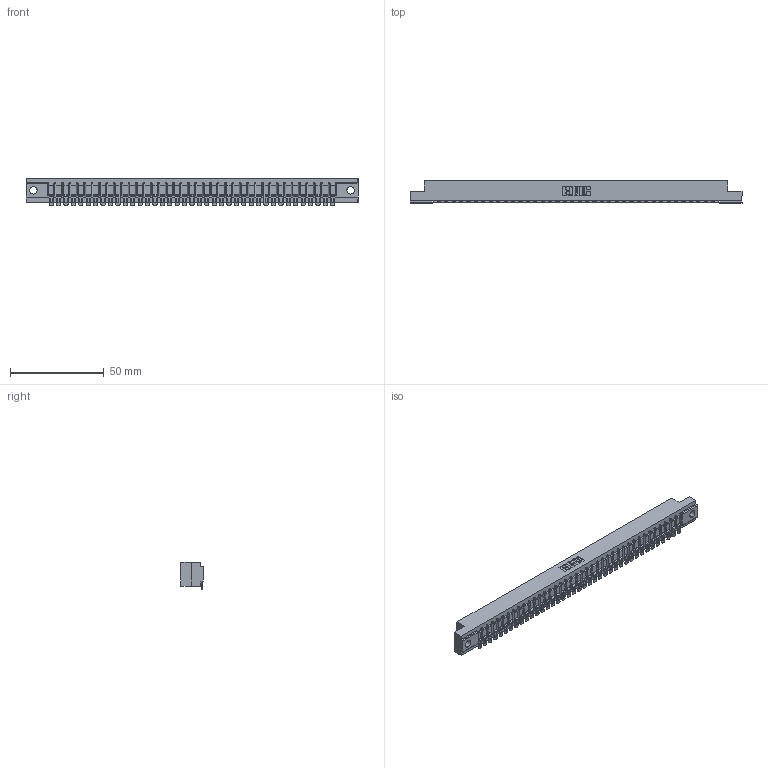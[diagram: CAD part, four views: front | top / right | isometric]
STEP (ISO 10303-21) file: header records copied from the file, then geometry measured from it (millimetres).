
FILE_DESCRIPTION (( 'STEP AP203' ), '1' );
FILE_NAME ('357-039-454-104.STEP', '2020-10-03T04:32:03', ( '' ), ( '' ), 'SwSTEP 2.0', 'SolidWorks 2020', '' );
FILE_SCHEMA (( 'CONFIG_CONTROL_DESIGN' ));
Length unit declared in the file: inch
Products named in the file (3): 357-039-454-104; 307-290-002_554; 307 Part_.156 Dia Mounting Holes
Assembly tree (40 placements, depth 2):
  357-039-454-104
    307 Part_.156 Dia Mounting Holes
    307-290-002_554  x39
Bounding box: 177.55 x 12.01 x 14.52 mm (x, y, z)
Volume: 18885.4 mm3; surface area: 23666 mm2
Topology: 40 solids, 40 shells, 3331 faces, 10226 edges, 6708 vertices
Faces by surface type: plane 1878, cylinder 1373, sphere 80
Entity records: 35187 total; most frequent: CARTESIAN_POINT 5940, ORIENTED_EDGE 5928, DIRECTION 5770, EDGE_CURVE 2964, VECTOR 2270, LINE 2270, VERTEX_POINT 1920, AXIS2_PLACEMENT_3D 1750
